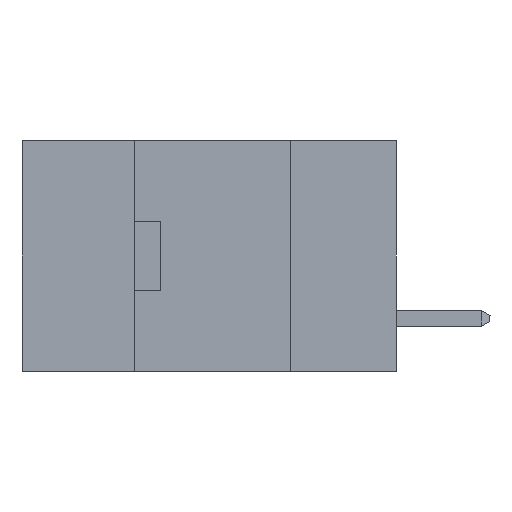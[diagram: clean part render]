
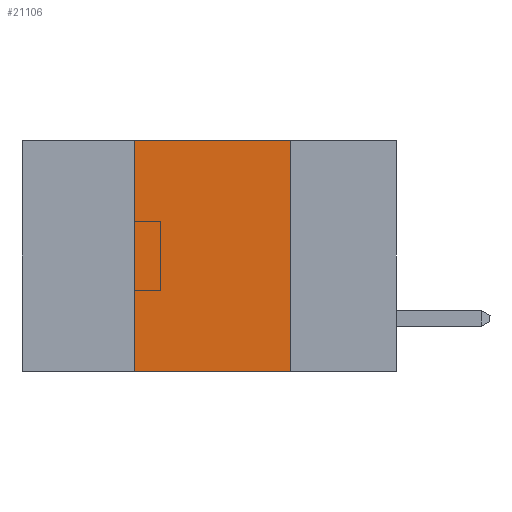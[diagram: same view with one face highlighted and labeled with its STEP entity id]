
A CAD part, left-side view. The second image highlights one B-rep face of the part: STEP entity #21106.
In plain terms, the highlighted planar face has unit normal (-1, 0, 0).
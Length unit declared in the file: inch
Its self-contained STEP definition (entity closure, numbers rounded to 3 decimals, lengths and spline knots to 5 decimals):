
#56 = LINE ( 'NONE', #7569, #22607 ) ;
#783 = CARTESIAN_POINT ( 'NONE',  ( 0., 0.42, 0. ) ) ;
#1031 = PLANE ( 'NONE',  #11863 ) ;
#1058 = CARTESIAN_POINT ( 'NONE',  ( 0., 0.6, -0.37 ) ) ;
#1248 = DIRECTION ( 'NONE',  ( 0., -1., 0. ) ) ;
#1922 = CARTESIAN_POINT ( 'NONE',  ( 0., 0.42, -0.37 ) ) ;
#2247 = VERTEX_POINT ( 'NONE', #783 ) ;
#3128 = DIRECTION ( 'NONE',  ( 0., 0., -1. ) ) ;
#5326 = CARTESIAN_POINT ( 'NONE',  ( 0., 0.42, -0.37 ) ) ;
#6128 = DIRECTION ( 'NONE',  ( 0., 0., 1. ) ) ;
#6966 = CARTESIAN_POINT ( 'NONE',  ( 0., 0.17, 0. ) ) ;
#7569 = CARTESIAN_POINT ( 'NONE',  ( 0., 0.6, 0. ) ) ;
#7690 = VECTOR ( 'NONE', #6128, 39.37008 ) ;
#8356 = LINE ( 'NONE', #1922, #7690 ) ;
#9536 = LINE ( 'NONE', #1058, #19072 ) ;
#9703 = ORIENTED_EDGE ( 'NONE', *, *, #26335, .F. ) ;
#10277 = VERTEX_POINT ( 'NONE', #6966 ) ;
#11863 = AXIS2_PLACEMENT_3D ( 'NONE', #21543, #15530, #3128 ) ;
#11901 = EDGE_CURVE ( 'NONE', #10277, #12392, #12707, .T. ) ;
#12001 = ORIENTED_EDGE ( 'NONE', *, *, #20464, .T. ) ;
#12392 = VERTEX_POINT ( 'NONE', #12826 ) ;
#12707 = LINE ( 'NONE', #21210, #17391 ) ;
#12826 = CARTESIAN_POINT ( 'NONE',  ( 0., 0.17, -0.37 ) ) ;
#13089 = EDGE_LOOP ( 'NONE', ( #14447, #13410, #9703, #12001 ) ) ;
#13410 = ORIENTED_EDGE ( 'NONE', *, *, #18225, .F. ) ;
#14007 = FACE_OUTER_BOUND ( 'NONE', #13089, .T. ) ;
#14447 = ORIENTED_EDGE ( 'NONE', *, *, #11901, .F. ) ;
#14805 = VERTEX_POINT ( 'NONE', #5326 ) ;
#15530 = DIRECTION ( 'NONE',  ( 1., 0., 0. ) ) ;
#17391 = VECTOR ( 'NONE', #19168, 39.37008 ) ;
#18225 = EDGE_CURVE ( 'NONE', #2247, #10277, #56, .T. ) ;
#19072 = VECTOR ( 'NONE', #25710, 39.37008 ) ;
#19168 = DIRECTION ( 'NONE',  ( 0., 0., -1. ) ) ;
#20464 = EDGE_CURVE ( 'NONE', #14805, #12392, #9536, .T. ) ;
#21106 = ADVANCED_FACE ( 'NONE', ( #14007 ), #1031, .F. ) ;
#21210 = CARTESIAN_POINT ( 'NONE',  ( 0., 0.17, -0.37 ) ) ;
#21543 = CARTESIAN_POINT ( 'NONE',  ( 0., 0.6, 0. ) ) ;
#22607 = VECTOR ( 'NONE', #1248, 39.37008 ) ;
#25710 = DIRECTION ( 'NONE',  ( 0., -1., 0. ) ) ;
#26335 = EDGE_CURVE ( 'NONE', #14805, #2247, #8356, .T. ) ;
